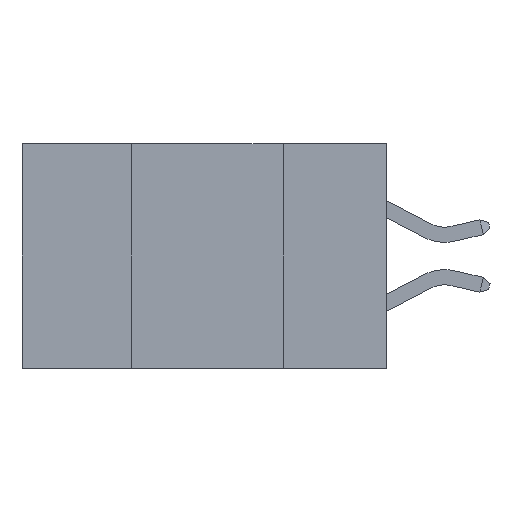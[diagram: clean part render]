
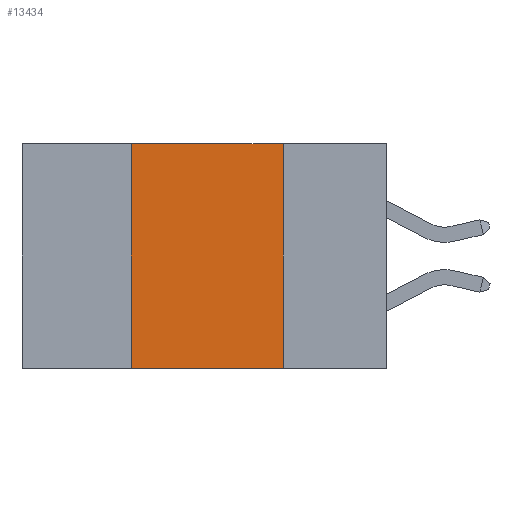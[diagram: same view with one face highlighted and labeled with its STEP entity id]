
A CAD part, left-side view. The second image highlights one B-rep face of the part: STEP entity #13434.
In plain terms, the highlighted planar face has unit normal (-1, 0, 0).
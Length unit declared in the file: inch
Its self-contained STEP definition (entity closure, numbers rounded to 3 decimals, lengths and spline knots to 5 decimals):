
#372 = VERTEX_POINT ( 'NONE', #12900 ) ;
#3165 = LINE ( 'NONE', #22915, #13598 ) ;
#5064 = CARTESIAN_POINT ( 'NONE',  ( 0., 0.6, 0. ) ) ;
#6852 = VERTEX_POINT ( 'NONE', #16886 ) ;
#8937 = VECTOR ( 'NONE', #21516, 39.37008 ) ;
#9163 = DIRECTION ( 'NONE',  ( 0., -1., 0. ) ) ;
#9676 = DIRECTION ( 'NONE',  ( 0., -1., 0. ) ) ;
#9761 = CARTESIAN_POINT ( 'NONE',  ( 0., 0.6, 0. ) ) ;
#10072 = ORIENTED_EDGE ( 'NONE', *, *, #14499, .F. ) ;
#10261 = ORIENTED_EDGE ( 'NONE', *, *, #22041, .T. ) ;
#11120 = VERTEX_POINT ( 'NONE', #17502 ) ;
#11566 = ORIENTED_EDGE ( 'NONE', *, *, #21280, .F. ) ;
#12138 = EDGE_LOOP ( 'NONE', ( #10072, #22620, #11566, #10261 ) ) ;
#12259 = DIRECTION ( 'NONE',  ( 1., 0., 0. ) ) ;
#12600 = CARTESIAN_POINT ( 'NONE',  ( 0., 0.17, 0. ) ) ;
#12900 = CARTESIAN_POINT ( 'NONE',  ( 0., 0.17, -0.37 ) ) ;
#13434 = ADVANCED_FACE ( 'NONE', ( #17231 ), #23486, .F. ) ;
#13598 = VECTOR ( 'NONE', #9163, 39.37008 ) ;
#14259 = DIRECTION ( 'NONE',  ( 0., 0., -1. ) ) ;
#14495 = AXIS2_PLACEMENT_3D ( 'NONE', #9761, #12259, #14259 ) ;
#14499 = EDGE_CURVE ( 'NONE', #11120, #372, #29373, .T. ) ;
#14881 = DIRECTION ( 'NONE',  ( 0., 0., -1. ) ) ;
#16886 = CARTESIAN_POINT ( 'NONE',  ( 0., 0.42, -0.37 ) ) ;
#17231 = FACE_OUTER_BOUND ( 'NONE', #12138, .T. ) ;
#17502 = CARTESIAN_POINT ( 'NONE',  ( 0., 0.17, 0. ) ) ;
#19245 = VECTOR ( 'NONE', #9676, 39.37008 ) ;
#19351 = LINE ( 'NONE', #20044, #8937 ) ;
#20044 = CARTESIAN_POINT ( 'NONE',  ( 0., 0.42, 0. ) ) ;
#21280 = EDGE_CURVE ( 'NONE', #6852, #25489, #19351, .T. ) ;
#21516 = DIRECTION ( 'NONE',  ( 0., 0., 1. ) ) ;
#22041 = EDGE_CURVE ( 'NONE', #6852, #372, #3165, .T. ) ;
#22597 = VECTOR ( 'NONE', #14881, 39.37008 ) ;
#22620 = ORIENTED_EDGE ( 'NONE', *, *, #29474, .F. ) ;
#22915 = CARTESIAN_POINT ( 'NONE',  ( 0., 0.6, -0.37 ) ) ;
#23486 = PLANE ( 'NONE',  #14495 ) ;
#25290 = LINE ( 'NONE', #5064, #19245 ) ;
#25489 = VERTEX_POINT ( 'NONE', #27131 ) ;
#27131 = CARTESIAN_POINT ( 'NONE',  ( 0., 0.42, 0. ) ) ;
#29373 = LINE ( 'NONE', #12600, #22597 ) ;
#29474 = EDGE_CURVE ( 'NONE', #25489, #11120, #25290, .T. ) ;
